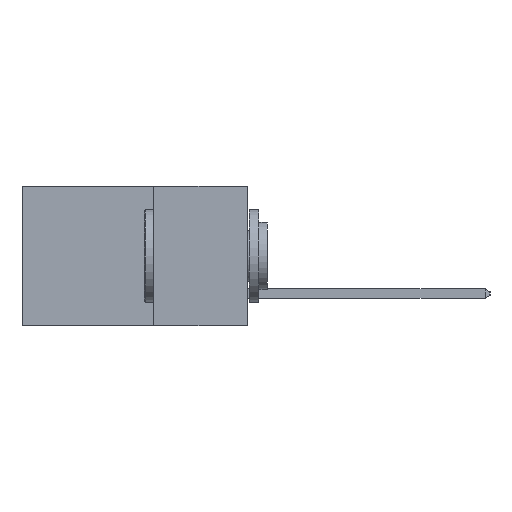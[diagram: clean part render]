
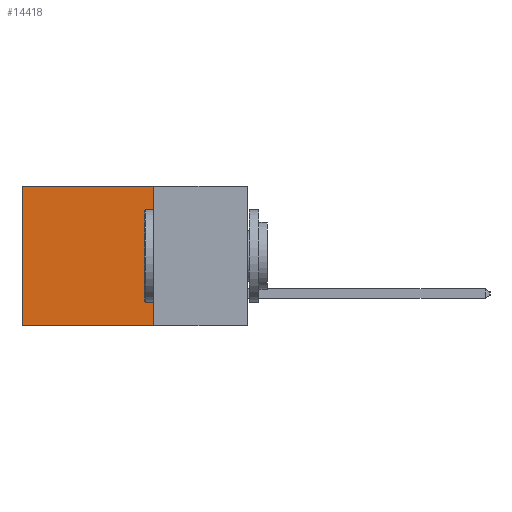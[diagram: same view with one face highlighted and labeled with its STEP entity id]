
A CAD part, left-side view. The second image highlights one B-rep face of the part: STEP entity #14418.
In plain terms, the highlighted planar face has unit normal (-1, 0, 0).
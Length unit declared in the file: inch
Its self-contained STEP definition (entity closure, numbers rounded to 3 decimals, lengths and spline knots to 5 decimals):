
#1383 = EDGE_LOOP ( 'NONE', ( #3731, #12346, #5051, #9363 ) ) ;
#1621 = CARTESIAN_POINT ( 'NONE',  ( 0.2615, 0.6, -0.37 ) ) ;
#1907 = CARTESIAN_POINT ( 'NONE',  ( 0.2615, 0.25, -0.37 ) ) ;
#1965 = DIRECTION ( 'NONE',  ( 0., 1., 0. ) ) ;
#2026 = EDGE_CURVE ( 'NONE', #5831, #15526, #3070, .T. ) ;
#2941 = VECTOR ( 'NONE', #6765, 39.37008 ) ;
#3070 = LINE ( 'NONE', #14257, #6373 ) ;
#3401 = VECTOR ( 'NONE', #1965, 39.37008 ) ;
#3433 = CARTESIAN_POINT ( 'NONE',  ( 0.2615, 0.25, 0. ) ) ;
#3721 = VERTEX_POINT ( 'NONE', #1621 ) ;
#3731 = ORIENTED_EDGE ( 'NONE', *, *, #15895, .T. ) ;
#5051 = ORIENTED_EDGE ( 'NONE', *, *, #11233, .F. ) ;
#5831 = VERTEX_POINT ( 'NONE', #3433 ) ;
#6373 = VECTOR ( 'NONE', #16679, 39.37008 ) ;
#6765 = DIRECTION ( 'NONE',  ( 0., 0., -1. ) ) ;
#7066 = DIRECTION ( 'NONE',  ( 0., 0., -1. ) ) ;
#7281 = AXIS2_PLACEMENT_3D ( 'NONE', #16566, #17911, #9606 ) ;
#8201 = CARTESIAN_POINT ( 'NONE',  ( 0.2615, 0.25, -0.37 ) ) ;
#9363 = ORIENTED_EDGE ( 'NONE', *, *, #2026, .T. ) ;
#9606 = DIRECTION ( 'NONE',  ( 0., 0., -1. ) ) ;
#10485 = LINE ( 'NONE', #13845, #2941 ) ;
#11233 = EDGE_CURVE ( 'NONE', #5831, #16579, #12677, .T. ) ;
#12346 = ORIENTED_EDGE ( 'NONE', *, *, #15502, .F. ) ;
#12677 = LINE ( 'NONE', #8201, #15961 ) ;
#13845 = CARTESIAN_POINT ( 'NONE',  ( 0.2615, 0.6, -0.37 ) ) ;
#14113 = FACE_OUTER_BOUND ( 'NONE', #1383, .T. ) ;
#14257 = CARTESIAN_POINT ( 'NONE',  ( 0.2615, 0.25, 0. ) ) ;
#14418 = ADVANCED_FACE ( 'NONE', ( #14113 ), #15226, .F. ) ;
#14720 = LINE ( 'NONE', #1907, #3401 ) ;
#15226 = PLANE ( 'NONE',  #7281 ) ;
#15502 = EDGE_CURVE ( 'NONE', #16579, #3721, #14720, .T. ) ;
#15526 = VERTEX_POINT ( 'NONE', #17459 ) ;
#15541 = CARTESIAN_POINT ( 'NONE',  ( 0.2615, 0.25, -0.37 ) ) ;
#15895 = EDGE_CURVE ( 'NONE', #15526, #3721, #10485, .T. ) ;
#15961 = VECTOR ( 'NONE', #7066, 39.37008 ) ;
#16566 = CARTESIAN_POINT ( 'NONE',  ( 0.2615, 0.25, -0.37 ) ) ;
#16579 = VERTEX_POINT ( 'NONE', #15541 ) ;
#16679 = DIRECTION ( 'NONE',  ( 0., 1., 0. ) ) ;
#17459 = CARTESIAN_POINT ( 'NONE',  ( 0.2615, 0.6, 0. ) ) ;
#17911 = DIRECTION ( 'NONE',  ( 1., 0., 0. ) ) ;
